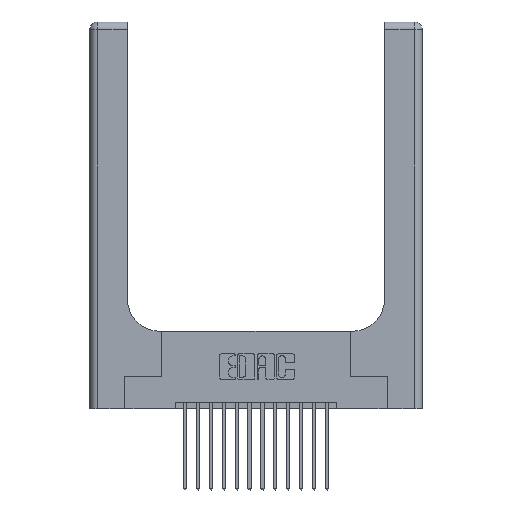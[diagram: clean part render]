
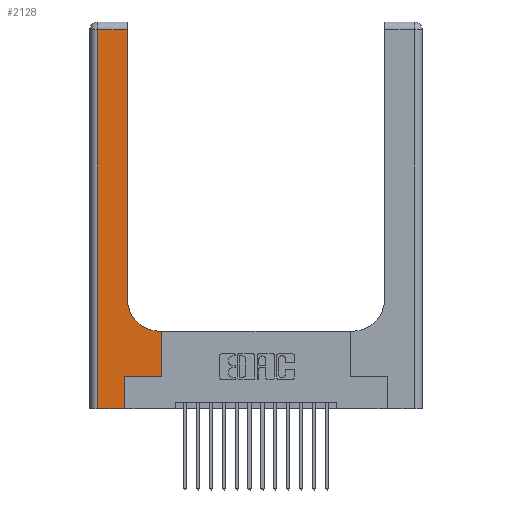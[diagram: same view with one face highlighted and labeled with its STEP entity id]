
A CAD part, top view. The second image highlights one B-rep face of the part: STEP entity #2128.
In plain terms, the highlighted planar face has unit normal (0, 0, 1).
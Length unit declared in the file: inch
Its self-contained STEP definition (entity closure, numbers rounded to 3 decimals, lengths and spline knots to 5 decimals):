
#18 = LINE ( 'NONE', #3153, #15046 ) ;
#354 = DIRECTION ( 'NONE',  ( -1., 0., 0. ) ) ;
#476 = CARTESIAN_POINT ( 'NONE',  ( 0.5415, 0.6, 0.37 ) ) ;
#802 = CARTESIAN_POINT ( 'NONE',  ( 0., 0., 0.37 ) ) ;
#818 = AXIS2_PLACEMENT_3D ( 'NONE', #13248, #13041, #12992 ) ;
#996 = CIRCLE ( 'NONE', #6895, 0.25 ) ;
#1391 = LINE ( 'NONE', #15256, #16258 ) ;
#1558 = VERTEX_POINT ( 'NONE', #3566 ) ;
#1721 = CARTESIAN_POINT ( 'NONE',  ( 0.269, 0., 0.37 ) ) ;
#1897 = DIRECTION ( 'NONE',  ( 1., 0., 0. ) ) ;
#2128 = ADVANCED_FACE ( 'NONE', ( #10043 ), #13080, .F. ) ;
#2499 = VERTEX_POINT ( 'NONE', #8612 ) ;
#2521 = VERTEX_POINT ( 'NONE', #8382 ) ;
#2840 = CARTESIAN_POINT ( 'NONE',  ( 0.06, 3., 0.37 ) ) ;
#2859 = ORIENTED_EDGE ( 'NONE', *, *, #8731, .T. ) ;
#3110 = ORIENTED_EDGE ( 'NONE', *, *, #18513, .T. ) ;
#3153 = CARTESIAN_POINT ( 'NONE',  ( 0.5585, 0.25, 0.37 ) ) ;
#3243 = LINE ( 'NONE', #802, #14686 ) ;
#3566 = CARTESIAN_POINT ( 'NONE',  ( 0.5585, 0.25, 0.37 ) ) ;
#3950 = DIRECTION ( 'NONE',  ( 0., 1., 0. ) ) ;
#4382 = CARTESIAN_POINT ( 'NONE',  ( 0.5415, 0.85, 0.37 ) ) ;
#4569 = ORIENTED_EDGE ( 'NONE', *, *, #8787, .T. ) ;
#5043 = ORIENTED_EDGE ( 'NONE', *, *, #15280, .T. ) ;
#5515 = ORIENTED_EDGE ( 'NONE', *, *, #16721, .T. ) ;
#5569 = EDGE_CURVE ( 'NONE', #11742, #18130, #1391, .T. ) ;
#5886 = DIRECTION ( 'NONE',  ( 1., 0., 0. ) ) ;
#6587 = CARTESIAN_POINT ( 'NONE',  ( 0., 2.94, 0.37 ) ) ;
#6895 = AXIS2_PLACEMENT_3D ( 'NONE', #4382, #14319, #5886 ) ;
#7070 = CARTESIAN_POINT ( 'NONE',  ( 0.2915, 3., 0.37 ) ) ;
#7938 = CARTESIAN_POINT ( 'NONE',  ( 0.2915, 0.6, 0.37 ) ) ;
#7975 = VECTOR ( 'NONE', #354, 39.37008 ) ;
#8277 = VERTEX_POINT ( 'NONE', #15352 ) ;
#8382 = CARTESIAN_POINT ( 'NONE',  ( 0.2915, 0.85, 0.37 ) ) ;
#8612 = CARTESIAN_POINT ( 'NONE',  ( 0.06, 0., 0.37 ) ) ;
#8731 = EDGE_CURVE ( 'NONE', #18130, #1558, #11231, .T. ) ;
#8787 = EDGE_CURVE ( 'NONE', #16586, #16275, #17701, .T. ) ;
#8895 = DIRECTION ( 'NONE',  ( 0., -1., 0. ) ) ;
#9564 = VECTOR ( 'NONE', #16793, 39.37008 ) ;
#9883 = EDGE_LOOP ( 'NONE', ( #16674, #4569, #5043, #5515, #17125, #2859, #11960, #13702, #3110 ) ) ;
#10025 = EDGE_CURVE ( 'NONE', #1558, #8277, #18, .T. ) ;
#10043 = FACE_OUTER_BOUND ( 'NONE', #9883, .T. ) ;
#10348 = VECTOR ( 'NONE', #12203, 39.37008 ) ;
#10558 = LINE ( 'NONE', #2840, #13376 ) ;
#10753 = CARTESIAN_POINT ( 'NONE',  ( 0.269, 0.25, 0.37 ) ) ;
#11159 = DIRECTION ( 'NONE',  ( 1., 0., 0. ) ) ;
#11231 = LINE ( 'NONE', #10753, #15757 ) ;
#11268 = LINE ( 'NONE', #7938, #7975 ) ;
#11742 = VERTEX_POINT ( 'NONE', #1721 ) ;
#11936 = VERTEX_POINT ( 'NONE', #476 ) ;
#11960 = ORIENTED_EDGE ( 'NONE', *, *, #10025, .T. ) ;
#12203 = DIRECTION ( 'NONE',  ( -1., 0., 0. ) ) ;
#12210 = CARTESIAN_POINT ( 'NONE',  ( 0.269, 0.25, 0.37 ) ) ;
#12736 = EDGE_CURVE ( 'NONE', #2521, #16586, #13257, .T. ) ;
#12992 = DIRECTION ( 'NONE',  ( -1., 0., 0. ) ) ;
#13041 = DIRECTION ( 'NONE',  ( 0., 0., -1. ) ) ;
#13080 = PLANE ( 'NONE',  #818 ) ;
#13248 = CARTESIAN_POINT ( 'NONE',  ( 0., 3., 0.37 ) ) ;
#13257 = LINE ( 'NONE', #7070, #9564 ) ;
#13376 = VECTOR ( 'NONE', #8895, 39.37008 ) ;
#13702 = ORIENTED_EDGE ( 'NONE', *, *, #16044, .T. ) ;
#14319 = DIRECTION ( 'NONE',  ( 0., 0., -1. ) ) ;
#14686 = VECTOR ( 'NONE', #11159, 39.37008 ) ;
#15046 = VECTOR ( 'NONE', #17399, 39.37008 ) ;
#15256 = CARTESIAN_POINT ( 'NONE',  ( 0.269, 0., 0.37 ) ) ;
#15280 = EDGE_CURVE ( 'NONE', #16275, #2499, #10558, .T. ) ;
#15352 = CARTESIAN_POINT ( 'NONE',  ( 0.5585, 0.6, 0.37 ) ) ;
#15757 = VECTOR ( 'NONE', #1897, 39.37008 ) ;
#16044 = EDGE_CURVE ( 'NONE', #8277, #11936, #11268, .T. ) ;
#16103 = CARTESIAN_POINT ( 'NONE',  ( 0.2915, 2.94, 0.37 ) ) ;
#16258 = VECTOR ( 'NONE', #3950, 39.37008 ) ;
#16275 = VERTEX_POINT ( 'NONE', #18117 ) ;
#16586 = VERTEX_POINT ( 'NONE', #16103 ) ;
#16674 = ORIENTED_EDGE ( 'NONE', *, *, #12736, .T. ) ;
#16721 = EDGE_CURVE ( 'NONE', #2499, #11742, #3243, .T. ) ;
#16793 = DIRECTION ( 'NONE',  ( 0., 1., 0. ) ) ;
#17125 = ORIENTED_EDGE ( 'NONE', *, *, #5569, .T. ) ;
#17399 = DIRECTION ( 'NONE',  ( 0., 1., 0. ) ) ;
#17701 = LINE ( 'NONE', #6587, #10348 ) ;
#18117 = CARTESIAN_POINT ( 'NONE',  ( 0.06, 2.94, 0.37 ) ) ;
#18130 = VERTEX_POINT ( 'NONE', #12210 ) ;
#18513 = EDGE_CURVE ( 'NONE', #11936, #2521, #996, .T. ) ;
